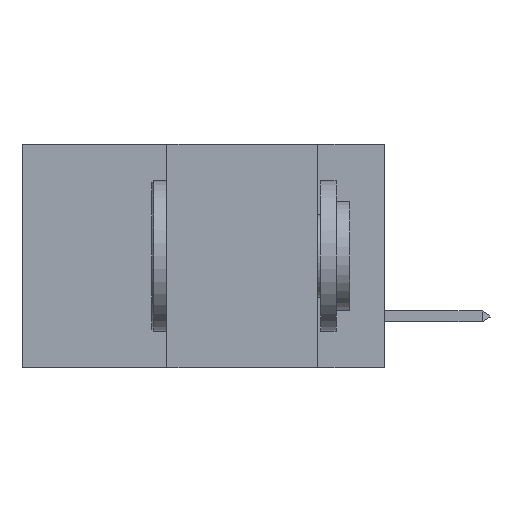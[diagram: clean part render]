
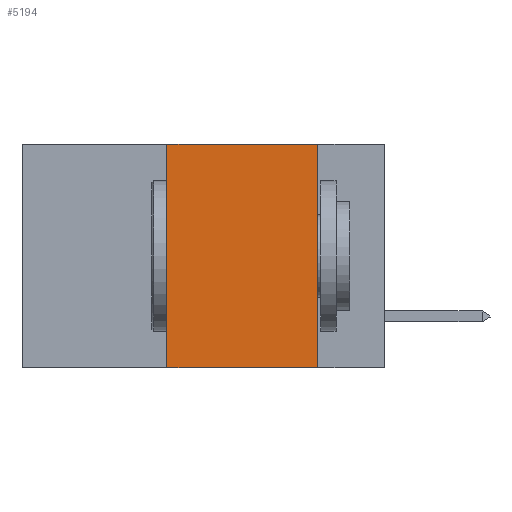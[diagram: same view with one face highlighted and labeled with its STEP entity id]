
A CAD part, left-side view. The second image highlights one B-rep face of the part: STEP entity #5194.
In plain terms, the highlighted planar face has unit normal (-1, 0, 0).
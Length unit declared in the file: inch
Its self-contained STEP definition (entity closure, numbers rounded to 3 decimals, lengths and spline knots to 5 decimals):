
#37 = CARTESIAN_POINT ( 'NONE',  ( 0., 0.36, 0. ) ) ;
#59 = DIRECTION ( 'NONE',  ( 0., 0., -1. ) ) ;
#80 = CARTESIAN_POINT ( 'NONE',  ( 0., 0.6, 0. ) ) ;
#128 = EDGE_LOOP ( 'NONE', ( #2976, #4765, #9003, #14195 ) ) ;
#644 = EDGE_CURVE ( 'NONE', #1868, #7352, #5908, .T. ) ;
#950 = VECTOR ( 'NONE', #7478, 39.37008 ) ;
#1254 = DIRECTION ( 'NONE',  ( 0., 0., -1. ) ) ;
#1578 = FACE_OUTER_BOUND ( 'NONE', #128, .T. ) ;
#1868 = VERTEX_POINT ( 'NONE', #11909 ) ;
#2456 = DIRECTION ( 'NONE',  ( 1., 0., 0. ) ) ;
#2635 = VECTOR ( 'NONE', #5871, 39.37008 ) ;
#2726 = VECTOR ( 'NONE', #1254, 39.37008 ) ;
#2873 = CARTESIAN_POINT ( 'NONE',  ( 0., 0.36, -0.37 ) ) ;
#2976 = ORIENTED_EDGE ( 'NONE', *, *, #12510, .F. ) ;
#4655 = CARTESIAN_POINT ( 'NONE',  ( 0., 0.6, -0.37 ) ) ;
#4765 = ORIENTED_EDGE ( 'NONE', *, *, #644, .F. ) ;
#5194 = ADVANCED_FACE ( 'NONE', ( #1578 ), #13506, .F. ) ;
#5205 = LINE ( 'NONE', #15844, #2726 ) ;
#5871 = DIRECTION ( 'NONE',  ( 0., -1., 0. ) ) ;
#5908 = LINE ( 'NONE', #80, #950 ) ;
#5922 = VECTOR ( 'NONE', #8667, 39.37008 ) ;
#7352 = VERTEX_POINT ( 'NONE', #8746 ) ;
#7478 = DIRECTION ( 'NONE',  ( 0., -1., 0. ) ) ;
#7506 = VERTEX_POINT ( 'NONE', #2873 ) ;
#7879 = EDGE_CURVE ( 'NONE', #7506, #1868, #12800, .T. ) ;
#8061 = CARTESIAN_POINT ( 'NONE',  ( 0., 0.11, -0.37 ) ) ;
#8667 = DIRECTION ( 'NONE',  ( 0., 0., 1. ) ) ;
#8746 = CARTESIAN_POINT ( 'NONE',  ( 0., 0.11, 0. ) ) ;
#8864 = VERTEX_POINT ( 'NONE', #8061 ) ;
#9003 = ORIENTED_EDGE ( 'NONE', *, *, #7879, .F. ) ;
#9110 = EDGE_CURVE ( 'NONE', #7506, #8864, #12552, .T. ) ;
#10827 = AXIS2_PLACEMENT_3D ( 'NONE', #14620, #2456, #59 ) ;
#11909 = CARTESIAN_POINT ( 'NONE',  ( 0., 0.36, 0. ) ) ;
#12510 = EDGE_CURVE ( 'NONE', #7352, #8864, #5205, .T. ) ;
#12552 = LINE ( 'NONE', #4655, #2635 ) ;
#12800 = LINE ( 'NONE', #37, #5922 ) ;
#13506 = PLANE ( 'NONE',  #10827 ) ;
#14195 = ORIENTED_EDGE ( 'NONE', *, *, #9110, .T. ) ;
#14620 = CARTESIAN_POINT ( 'NONE',  ( 0., 0.6, 0. ) ) ;
#15844 = CARTESIAN_POINT ( 'NONE',  ( 0., 0.11, 0. ) ) ;
